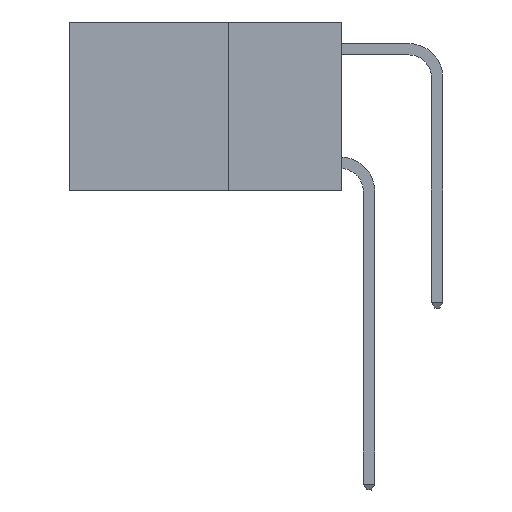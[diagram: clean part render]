
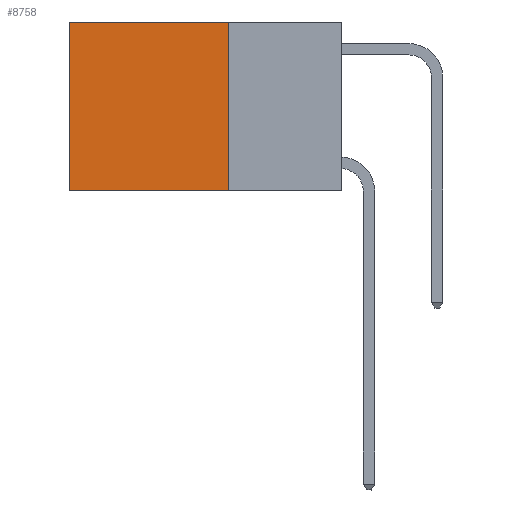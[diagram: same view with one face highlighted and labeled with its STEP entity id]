
A CAD part, left-side view. The second image highlights one B-rep face of the part: STEP entity #8758.
In plain terms, the highlighted planar face has unit normal (-1, 0, 0).
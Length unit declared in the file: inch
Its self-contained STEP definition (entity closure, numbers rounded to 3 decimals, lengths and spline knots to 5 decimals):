
#1359 = DIRECTION ( 'NONE',  ( 0., 0., -1. ) ) ;
#1708 = VECTOR ( 'NONE', #8249, 39.37008 ) ;
#1969 = DIRECTION ( 'NONE',  ( 0., 1., 0. ) ) ;
#3153 = VECTOR ( 'NONE', #1969, 39.37008 ) ;
#4171 = CARTESIAN_POINT ( 'NONE',  ( 0.2625, 0.25, 0. ) ) ;
#4376 = EDGE_LOOP ( 'NONE', ( #6582, #16366, #21237, #19256 ) ) ;
#4915 = VERTEX_POINT ( 'NONE', #11017 ) ;
#5193 = EDGE_CURVE ( 'NONE', #9499, #7931, #20746, .T. ) ;
#6582 = ORIENTED_EDGE ( 'NONE', *, *, #19050, .T. ) ;
#7390 = PLANE ( 'NONE',  #16521 ) ;
#7931 = VERTEX_POINT ( 'NONE', #12801 ) ;
#8249 = DIRECTION ( 'NONE',  ( 0., 1., 0. ) ) ;
#8758 = ADVANCED_FACE ( 'NONE', ( #19026 ), #7390, .F. ) ;
#9148 = DIRECTION ( 'NONE',  ( 0., 0., -1. ) ) ;
#9195 = EDGE_CURVE ( 'NONE', #9499, #12987, #11125, .T. ) ;
#9499 = VERTEX_POINT ( 'NONE', #4171 ) ;
#10079 = VECTOR ( 'NONE', #1359, 39.37008 ) ;
#10587 = VECTOR ( 'NONE', #13729, 39.37008 ) ;
#10663 = CARTESIAN_POINT ( 'NONE',  ( 0.2625, 0.25, -0.37 ) ) ;
#11017 = CARTESIAN_POINT ( 'NONE',  ( 0.2625, 0.6, -0.37 ) ) ;
#11125 = LINE ( 'NONE', #12004, #10587 ) ;
#11745 = LINE ( 'NONE', #15311, #10079 ) ;
#12004 = CARTESIAN_POINT ( 'NONE',  ( 0.2625, 0.25, 0. ) ) ;
#12445 = LINE ( 'NONE', #10663, #3153 ) ;
#12801 = CARTESIAN_POINT ( 'NONE',  ( 0.2625, 0.6, 0. ) ) ;
#12987 = VERTEX_POINT ( 'NONE', #21382 ) ;
#13729 = DIRECTION ( 'NONE',  ( 0., 0., -1. ) ) ;
#15311 = CARTESIAN_POINT ( 'NONE',  ( 0.2625, 0.6, 0. ) ) ;
#16366 = ORIENTED_EDGE ( 'NONE', *, *, #20609, .F. ) ;
#16521 = AXIS2_PLACEMENT_3D ( 'NONE', #17822, #19560, #9148 ) ;
#17822 = CARTESIAN_POINT ( 'NONE',  ( 0.2625, 0.25, 0. ) ) ;
#19026 = FACE_OUTER_BOUND ( 'NONE', #4376, .T. ) ;
#19050 = EDGE_CURVE ( 'NONE', #7931, #4915, #11745, .T. ) ;
#19256 = ORIENTED_EDGE ( 'NONE', *, *, #5193, .T. ) ;
#19560 = DIRECTION ( 'NONE',  ( 1., 0., 0. ) ) ;
#20415 = CARTESIAN_POINT ( 'NONE',  ( 0.2625, 0.25, 0. ) ) ;
#20609 = EDGE_CURVE ( 'NONE', #12987, #4915, #12445, .T. ) ;
#20746 = LINE ( 'NONE', #20415, #1708 ) ;
#21237 = ORIENTED_EDGE ( 'NONE', *, *, #9195, .F. ) ;
#21382 = CARTESIAN_POINT ( 'NONE',  ( 0.2625, 0.25, -0.37 ) ) ;
